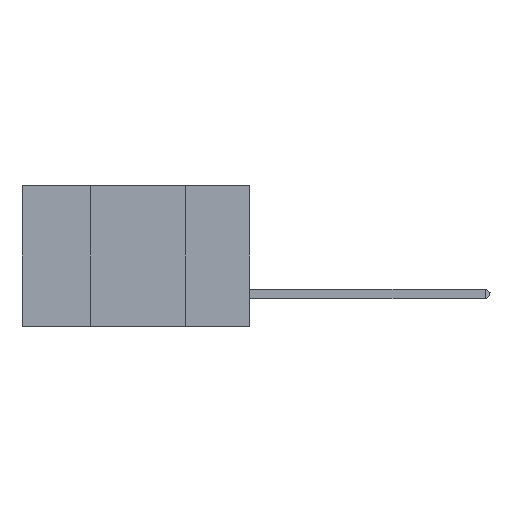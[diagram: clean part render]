
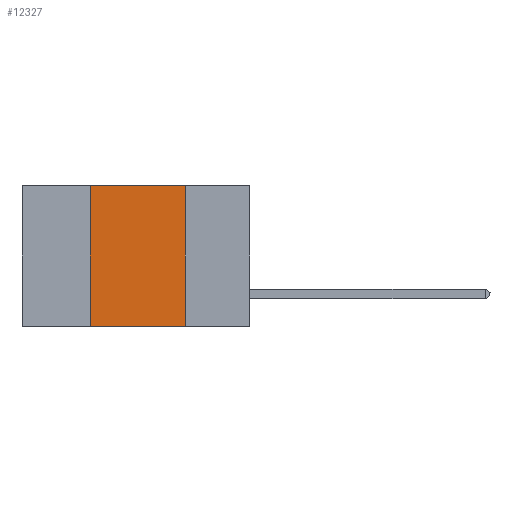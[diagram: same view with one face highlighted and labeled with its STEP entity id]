
A CAD part, left-side view. The second image highlights one B-rep face of the part: STEP entity #12327.
In plain terms, the highlighted planar face has unit normal (-1, 0, 0).
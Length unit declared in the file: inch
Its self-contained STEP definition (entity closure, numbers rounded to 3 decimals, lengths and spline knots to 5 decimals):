
#2558 = VERTEX_POINT ( 'NONE', #8978 ) ;
#3895 = VECTOR ( 'NONE', #26630, 39.37008 ) ;
#4198 = VECTOR ( 'NONE', #10077, 39.37008 ) ;
#6846 = VECTOR ( 'NONE', #28373, 39.37008 ) ;
#7072 = VECTOR ( 'NONE', #21261, 39.37008 ) ;
#8978 = CARTESIAN_POINT ( 'NONE',  ( 0., 0.17, 0. ) ) ;
#10077 = DIRECTION ( 'NONE',  ( 0., 0., -1. ) ) ;
#11457 = EDGE_LOOP ( 'NONE', ( #18178, #11941, #24284, #14984 ) ) ;
#11941 = ORIENTED_EDGE ( 'NONE', *, *, #16939, .F. ) ;
#12327 = ADVANCED_FACE ( 'NONE', ( #28961 ), #25523, .F. ) ;
#13084 = VERTEX_POINT ( 'NONE', #20470 ) ;
#13167 = VERTEX_POINT ( 'NONE', #25810 ) ;
#14439 = CARTESIAN_POINT ( 'NONE',  ( 0., 0.6, 0. ) ) ;
#14597 = EDGE_CURVE ( 'NONE', #13167, #13084, #17468, .T. ) ;
#14980 = CARTESIAN_POINT ( 'NONE',  ( 0., 0.42, 0. ) ) ;
#14984 = ORIENTED_EDGE ( 'NONE', *, *, #33392, .T. ) ;
#16939 = EDGE_CURVE ( 'NONE', #13084, #2558, #26276, .T. ) ;
#17468 = LINE ( 'NONE', #14980, #3895 ) ;
#18178 = ORIENTED_EDGE ( 'NONE', *, *, #29410, .F. ) ;
#20470 = CARTESIAN_POINT ( 'NONE',  ( 0., 0.42, 0. ) ) ;
#21261 = DIRECTION ( 'NONE',  ( 0., -1., 0. ) ) ;
#21532 = CARTESIAN_POINT ( 'NONE',  ( 0., 0.17, 0. ) ) ;
#21888 = AXIS2_PLACEMENT_3D ( 'NONE', #14439, #26094, #37750 ) ;
#24284 = ORIENTED_EDGE ( 'NONE', *, *, #14597, .F. ) ;
#24952 = LINE ( 'NONE', #21532, #4198 ) ;
#25523 = PLANE ( 'NONE',  #21888 ) ;
#25810 = CARTESIAN_POINT ( 'NONE',  ( 0., 0.42, -0.37 ) ) ;
#26094 = DIRECTION ( 'NONE',  ( 1., 0., 0. ) ) ;
#26276 = LINE ( 'NONE', #28764, #7072 ) ;
#26630 = DIRECTION ( 'NONE',  ( 0., 0., 1. ) ) ;
#28373 = DIRECTION ( 'NONE',  ( 0., -1., 0. ) ) ;
#28764 = CARTESIAN_POINT ( 'NONE',  ( 0., 0.6, 0. ) ) ;
#28961 = FACE_OUTER_BOUND ( 'NONE', #11457, .T. ) ;
#29410 = EDGE_CURVE ( 'NONE', #2558, #36064, #24952, .T. ) ;
#31422 = LINE ( 'NONE', #35057, #6846 ) ;
#32063 = CARTESIAN_POINT ( 'NONE',  ( 0., 0.17, -0.37 ) ) ;
#33392 = EDGE_CURVE ( 'NONE', #13167, #36064, #31422, .T. ) ;
#35057 = CARTESIAN_POINT ( 'NONE',  ( 0., 0.6, -0.37 ) ) ;
#36064 = VERTEX_POINT ( 'NONE', #32063 ) ;
#37750 = DIRECTION ( 'NONE',  ( 0., 0., -1. ) ) ;
